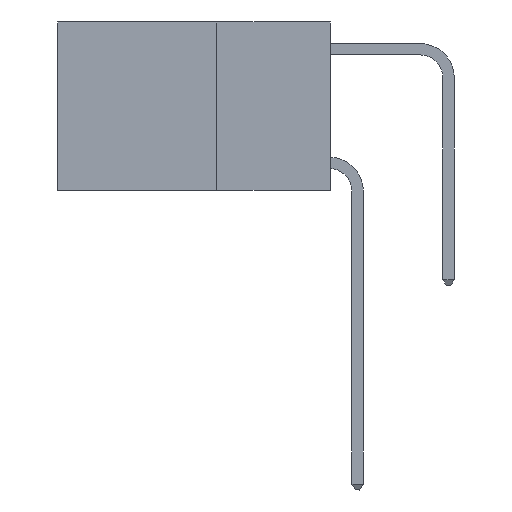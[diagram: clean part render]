
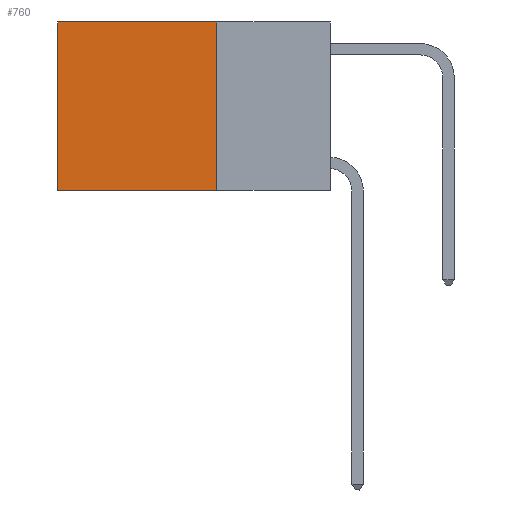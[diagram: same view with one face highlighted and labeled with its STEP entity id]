
A CAD part, left-side view. The second image highlights one B-rep face of the part: STEP entity #760.
In plain terms, the highlighted planar face has unit normal (-1, 0, 0).
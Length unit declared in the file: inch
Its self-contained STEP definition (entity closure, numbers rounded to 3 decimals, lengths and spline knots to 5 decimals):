
#155 = ORIENTED_EDGE ( 'NONE', *, *, #10365, .F. ) ;
#760 = ADVANCED_FACE ( 'NONE', ( #23027 ), #1554, .F. ) ;
#833 = CARTESIAN_POINT ( 'NONE',  ( 0.2625, 0.25, -0.37 ) ) ;
#844 = EDGE_LOOP ( 'NONE', ( #12183, #155, #15622, #2449 ) ) ;
#1554 = PLANE ( 'NONE',  #20956 ) ;
#2449 = ORIENTED_EDGE ( 'NONE', *, *, #14381, .T. ) ;
#2497 = EDGE_CURVE ( 'NONE', #23704, #6655, #20475, .T. ) ;
#3501 = EDGE_CURVE ( 'NONE', #11707, #6335, #24794, .T. ) ;
#3549 = DIRECTION ( 'NONE',  ( 0., 0., -1. ) ) ;
#4495 = VECTOR ( 'NONE', #5799, 39.37008 ) ;
#5125 = LINE ( 'NONE', #11558, #4495 ) ;
#5682 = DIRECTION ( 'NONE',  ( 0., 0., -1. ) ) ;
#5799 = DIRECTION ( 'NONE',  ( 0., 1., 0. ) ) ;
#6335 = VERTEX_POINT ( 'NONE', #24906 ) ;
#6655 = VERTEX_POINT ( 'NONE', #833 ) ;
#8538 = DIRECTION ( 'NONE',  ( 0., 1., 0. ) ) ;
#8823 = CARTESIAN_POINT ( 'NONE',  ( 0.2625, 0.25, 0. ) ) ;
#10365 = EDGE_CURVE ( 'NONE', #6655, #6335, #12980, .T. ) ;
#10803 = CARTESIAN_POINT ( 'NONE',  ( 0.2625, 0.25, 0. ) ) ;
#11558 = CARTESIAN_POINT ( 'NONE',  ( 0.2625, 0.25, 0. ) ) ;
#11707 = VERTEX_POINT ( 'NONE', #24005 ) ;
#12183 = ORIENTED_EDGE ( 'NONE', *, *, #3501, .T. ) ;
#12980 = LINE ( 'NONE', #20339, #18245 ) ;
#14276 = VECTOR ( 'NONE', #5682, 39.37008 ) ;
#14381 = EDGE_CURVE ( 'NONE', #23704, #11707, #5125, .T. ) ;
#15212 = VECTOR ( 'NONE', #22652, 39.37008 ) ;
#15368 = DIRECTION ( 'NONE',  ( 1., 0., 0. ) ) ;
#15622 = ORIENTED_EDGE ( 'NONE', *, *, #2497, .F. ) ;
#18245 = VECTOR ( 'NONE', #8538, 39.37008 ) ;
#19466 = CARTESIAN_POINT ( 'NONE',  ( 0.2625, 0.6, 0. ) ) ;
#20339 = CARTESIAN_POINT ( 'NONE',  ( 0.2625, 0.25, -0.37 ) ) ;
#20475 = LINE ( 'NONE', #10803, #15212 ) ;
#20956 = AXIS2_PLACEMENT_3D ( 'NONE', #21259, #15368, #3549 ) ;
#21259 = CARTESIAN_POINT ( 'NONE',  ( 0.2625, 0.25, 0. ) ) ;
#22652 = DIRECTION ( 'NONE',  ( 0., 0., -1. ) ) ;
#23027 = FACE_OUTER_BOUND ( 'NONE', #844, .T. ) ;
#23704 = VERTEX_POINT ( 'NONE', #8823 ) ;
#24005 = CARTESIAN_POINT ( 'NONE',  ( 0.2625, 0.6, 0. ) ) ;
#24794 = LINE ( 'NONE', #19466, #14276 ) ;
#24906 = CARTESIAN_POINT ( 'NONE',  ( 0.2625, 0.6, -0.37 ) ) ;
